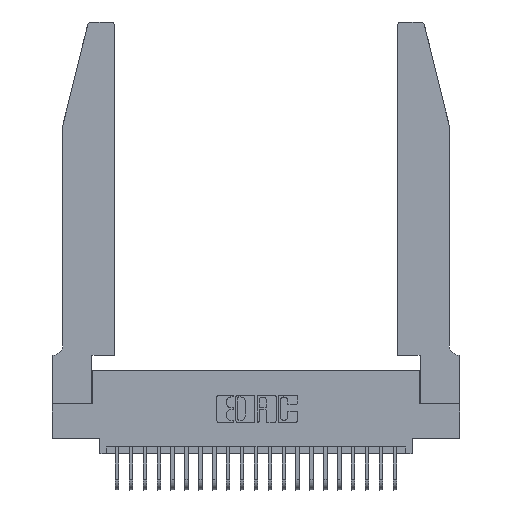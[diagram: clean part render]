
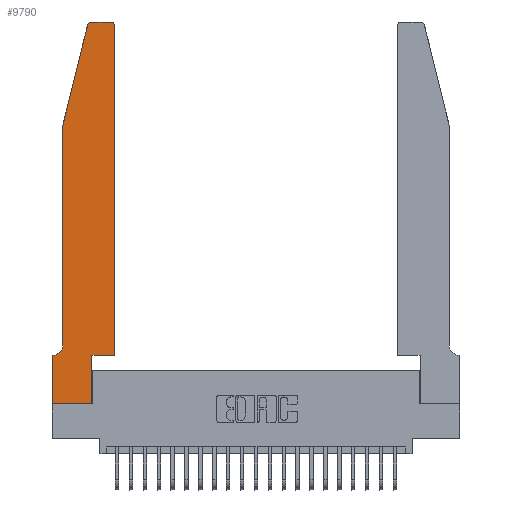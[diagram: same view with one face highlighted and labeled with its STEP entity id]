
A CAD part, top view. The second image highlights one B-rep face of the part: STEP entity #9790.
In plain terms, the highlighted planar face has unit normal (0, 0, 1).
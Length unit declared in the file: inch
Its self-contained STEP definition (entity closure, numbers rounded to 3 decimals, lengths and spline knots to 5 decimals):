
#352 = CARTESIAN_POINT ( 'NONE',  ( 0.284, 2.75, 0.37 ) ) ;
#439 = VECTOR ( 'NONE', #3185, 39.37008 ) ;
#571 = ORIENTED_EDGE ( 'NONE', *, *, #16472, .T. ) ;
#606 = ORIENTED_EDGE ( 'NONE', *, *, #23239, .T. ) ;
#646 = CARTESIAN_POINT ( 'NONE',  ( 0.0055, 0.42, 0.37 ) ) ;
#878 = ORIENTED_EDGE ( 'NONE', *, *, #8877, .T. ) ;
#970 = CARTESIAN_POINT ( 'NONE',  ( 0.0755, 0.42, 0.37 ) ) ;
#1180 = DIRECTION ( 'NONE',  ( 1., 0., 0. ) ) ;
#1200 = VERTEX_POINT ( 'NONE', #5058 ) ;
#1417 = ORIENTED_EDGE ( 'NONE', *, *, #19969, .T. ) ;
#1631 = FACE_OUTER_BOUND ( 'NONE', #4261, .T. ) ;
#1677 = LINE ( 'NONE', #14200, #6096 ) ;
#1933 = ORIENTED_EDGE ( 'NONE', *, *, #22181, .T. ) ;
#1976 = ORIENTED_EDGE ( 'NONE', *, *, #5741, .T. ) ;
#2213 = ORIENTED_EDGE ( 'NONE', *, *, #19166, .T. ) ;
#2580 = DIRECTION ( 'NONE',  ( -1., 0., 0. ) ) ;
#2696 = CARTESIAN_POINT ( 'NONE',  ( 0., 0., 0.37 ) ) ;
#2806 = DIRECTION ( 'NONE',  ( 1., 0., 0. ) ) ;
#3185 = DIRECTION ( 'NONE',  ( -0.239, -0.971, 0. ) ) ;
#3774 = VERTEX_POINT ( 'NONE', #2696 ) ;
#3804 = LINE ( 'NONE', #17969, #22472 ) ;
#4261 = EDGE_LOOP ( 'NONE', ( #1417, #1976, #1933, #878, #2213, #17485, #5046, #14057, #12267, #571, #606, #12116 ) ) ;
#4417 = LINE ( 'NONE', #14027, #12931 ) ;
#4482 = CARTESIAN_POINT ( 'NONE',  ( 0.4505, 0.35, 0.37 ) ) ;
#4497 = CIRCLE ( 'NONE', #11994, 0.03 ) ;
#4889 = LINE ( 'NONE', #14094, #439 ) ;
#4948 = LINE ( 'NONE', #9753, #23013 ) ;
#4957 = EDGE_CURVE ( 'NONE', #8138, #17568, #17290, .T. ) ;
#5046 = ORIENTED_EDGE ( 'NONE', *, *, #8492, .T. ) ;
#5053 = DIRECTION ( 'NONE',  ( 1., 0., 0. ) ) ;
#5058 = CARTESIAN_POINT ( 'NONE',  ( 0.25487, 2.72718, 0.37 ) ) ;
#5741 = EDGE_CURVE ( 'NONE', #21868, #1200, #4497, .T. ) ;
#6096 = VECTOR ( 'NONE', #7123, 39.37008 ) ;
#6304 = VECTOR ( 'NONE', #15810, 39.37008 ) ;
#6313 = DIRECTION ( 'NONE',  ( 0., 0., 1. ) ) ;
#6400 = CARTESIAN_POINT ( 'NONE',  ( 0.4505, 2.72, 0.37 ) ) ;
#7123 = DIRECTION ( 'NONE',  ( 0., -1., 0. ) ) ;
#7156 = VECTOR ( 'NONE', #19096, 39.37008 ) ;
#7190 = DIRECTION ( 'NONE',  ( 1., 0., 0. ) ) ;
#7473 = LINE ( 'NONE', #12252, #6304 ) ;
#8138 = VERTEX_POINT ( 'NONE', #14155 ) ;
#8319 = CARTESIAN_POINT ( 'NONE',  ( 0., 0.35, 0.37 ) ) ;
#8492 = EDGE_CURVE ( 'NONE', #17568, #3774, #4948, .T. ) ;
#8621 = VERTEX_POINT ( 'NONE', #22689 ) ;
#8877 = EDGE_CURVE ( 'NONE', #19451, #19281, #1677, .T. ) ;
#9753 = CARTESIAN_POINT ( 'NONE',  ( 0., 0., 0.37 ) ) ;
#9790 = ADVANCED_FACE ( 'NONE', ( #1631 ), #11926, .T. ) ;
#9924 = LINE ( 'NONE', #21318, #18937 ) ;
#10113 = CARTESIAN_POINT ( 'NONE',  ( 0.0755, 0.35, 0.37 ) ) ;
#10115 = CARTESIAN_POINT ( 'NONE',  ( 0., 0.35, 0.37 ) ) ;
#10983 = CIRCLE ( 'NONE', #15241, 0.07 ) ;
#11926 = PLANE ( 'NONE',  #21099 ) ;
#11994 = AXIS2_PLACEMENT_3D ( 'NONE', #22967, #12203, #1180 ) ;
#12116 = ORIENTED_EDGE ( 'NONE', *, *, #16836, .T. ) ;
#12203 = DIRECTION ( 'NONE',  ( 0., 0., 1. ) ) ;
#12252 = CARTESIAN_POINT ( 'NONE',  ( 0.2865, 0.35, 0.37 ) ) ;
#12267 = ORIENTED_EDGE ( 'NONE', *, *, #22744, .T. ) ;
#12931 = VECTOR ( 'NONE', #17584, 39.37008 ) ;
#13515 = DIRECTION ( 'NONE',  ( 0., 0., -1. ) ) ;
#13717 = DIRECTION ( 'NONE',  ( 0., 0., 1. ) ) ;
#14027 = CARTESIAN_POINT ( 'NONE',  ( 0.2605, 2.75, 0.37 ) ) ;
#14057 = ORIENTED_EDGE ( 'NONE', *, *, #18358, .T. ) ;
#14094 = CARTESIAN_POINT ( 'NONE',  ( 0.0755, 2., 0.37 ) ) ;
#14155 = CARTESIAN_POINT ( 'NONE',  ( 0.0055, 0.35, 0.37 ) ) ;
#14192 = VECTOR ( 'NONE', #20776, 39.37008 ) ;
#14200 = CARTESIAN_POINT ( 'NONE',  ( 0.0755, 2., 0.37 ) ) ;
#14404 = CARTESIAN_POINT ( 'NONE',  ( 0.2865, 0., 0.37 ) ) ;
#14604 = CARTESIAN_POINT ( 'NONE',  ( 0.4505, 0.35, 0.37 ) ) ;
#14765 = LINE ( 'NONE', #4482, #14192 ) ;
#15154 = VERTEX_POINT ( 'NONE', #6400 ) ;
#15241 = AXIS2_PLACEMENT_3D ( 'NONE', #646, #13515, #2580 ) ;
#15810 = DIRECTION ( 'NONE',  ( 0., 1., 0. ) ) ;
#16384 = CIRCLE ( 'NONE', #19695, 0.03 ) ;
#16472 = EDGE_CURVE ( 'NONE', #8621, #19581, #9924, .T. ) ;
#16836 = EDGE_CURVE ( 'NONE', #15154, #17085, #16384, .T. ) ;
#17085 = VERTEX_POINT ( 'NONE', #19646 ) ;
#17129 = CARTESIAN_POINT ( 'NONE',  ( 0.4205, 2.72, 0.37 ) ) ;
#17290 = LINE ( 'NONE', #10113, #7156 ) ;
#17485 = ORIENTED_EDGE ( 'NONE', *, *, #4957, .T. ) ;
#17568 = VERTEX_POINT ( 'NONE', #8319 ) ;
#17584 = DIRECTION ( 'NONE',  ( -1., 0., 0. ) ) ;
#17969 = CARTESIAN_POINT ( 'NONE',  ( 0., 0., 0.37 ) ) ;
#18358 = EDGE_CURVE ( 'NONE', #3774, #22290, #3804, .T. ) ;
#18937 = VECTOR ( 'NONE', #5053, 39.37008 ) ;
#18954 = DIRECTION ( 'NONE',  ( 1., 0., 0. ) ) ;
#19096 = DIRECTION ( 'NONE',  ( -1., 0., 0. ) ) ;
#19166 = EDGE_CURVE ( 'NONE', #19281, #8138, #10983, .T. ) ;
#19281 = VERTEX_POINT ( 'NONE', #970 ) ;
#19451 = VERTEX_POINT ( 'NONE', #21456 ) ;
#19581 = VERTEX_POINT ( 'NONE', #14604 ) ;
#19646 = CARTESIAN_POINT ( 'NONE',  ( 0.4205, 2.75, 0.37 ) ) ;
#19695 = AXIS2_PLACEMENT_3D ( 'NONE', #17129, #6313, #18954 ) ;
#19969 = EDGE_CURVE ( 'NONE', #17085, #21868, #4417, .T. ) ;
#20776 = DIRECTION ( 'NONE',  ( 0., 1., 0. ) ) ;
#21099 = AXIS2_PLACEMENT_3D ( 'NONE', #10115, #13717, #2806 ) ;
#21318 = CARTESIAN_POINT ( 'NONE',  ( 0.4505, 0.35, 0.37 ) ) ;
#21456 = CARTESIAN_POINT ( 'NONE',  ( 0.0755, 2., 0.37 ) ) ;
#21868 = VERTEX_POINT ( 'NONE', #352 ) ;
#22181 = EDGE_CURVE ( 'NONE', #1200, #19451, #4889, .T. ) ;
#22290 = VERTEX_POINT ( 'NONE', #14404 ) ;
#22330 = DIRECTION ( 'NONE',  ( 0., -1., 0. ) ) ;
#22472 = VECTOR ( 'NONE', #7190, 39.37008 ) ;
#22689 = CARTESIAN_POINT ( 'NONE',  ( 0.2865, 0.35, 0.37 ) ) ;
#22744 = EDGE_CURVE ( 'NONE', #22290, #8621, #7473, .T. ) ;
#22967 = CARTESIAN_POINT ( 'NONE',  ( 0.284, 2.72, 0.37 ) ) ;
#23013 = VECTOR ( 'NONE', #22330, 39.37008 ) ;
#23239 = EDGE_CURVE ( 'NONE', #19581, #15154, #14765, .T. ) ;
